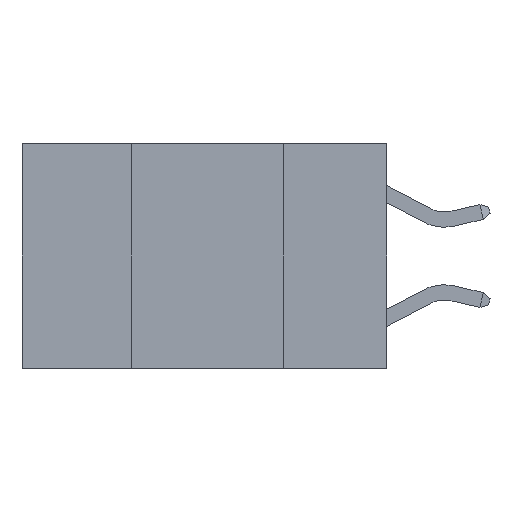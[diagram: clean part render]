
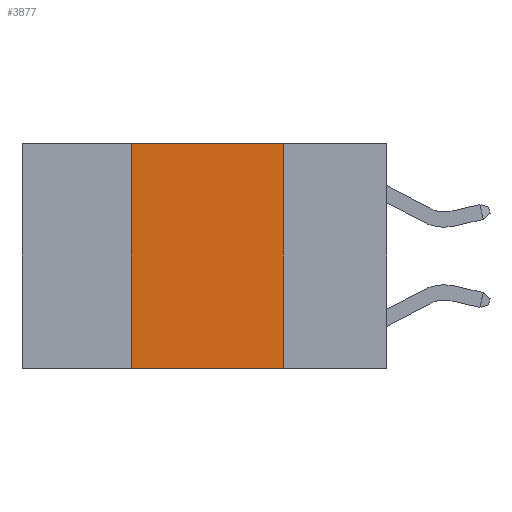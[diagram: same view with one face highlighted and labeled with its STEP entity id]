
A CAD part, left-side view. The second image highlights one B-rep face of the part: STEP entity #3877.
In plain terms, the highlighted planar face has unit normal (-1, 0, 0).
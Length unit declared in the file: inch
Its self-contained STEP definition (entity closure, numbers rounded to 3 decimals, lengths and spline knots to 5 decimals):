
#392 = VERTEX_POINT ( 'NONE', #10658 ) ;
#1095 = EDGE_LOOP ( 'NONE', ( #10278, #11160, #5317, #4137 ) ) ;
#2030 = CARTESIAN_POINT ( 'NONE',  ( 0., 0.42, 0. ) ) ;
#2975 = VECTOR ( 'NONE', #8717, 39.37008 ) ;
#3010 = CARTESIAN_POINT ( 'NONE',  ( 0., 0.6, 0. ) ) ;
#3042 = EDGE_CURVE ( 'NONE', #7221, #392, #9902, .T. ) ;
#3664 = CARTESIAN_POINT ( 'NONE',  ( 0., 0.6, -0.37 ) ) ;
#3715 = LINE ( 'NONE', #2030, #9602 ) ;
#3800 = DIRECTION ( 'NONE',  ( 1., 0., 0. ) ) ;
#3877 = ADVANCED_FACE ( 'NONE', ( #3980 ), #8273, .F. ) ;
#3980 = FACE_OUTER_BOUND ( 'NONE', #1095, .T. ) ;
#4137 = ORIENTED_EDGE ( 'NONE', *, *, #3042, .T. ) ;
#4946 = EDGE_CURVE ( 'NONE', #7221, #8030, #3715, .T. ) ;
#5032 = CARTESIAN_POINT ( 'NONE',  ( 0., 0.17, 0. ) ) ;
#5317 = ORIENTED_EDGE ( 'NONE', *, *, #4946, .F. ) ;
#5412 = CARTESIAN_POINT ( 'NONE',  ( 0., 0.42, 0. ) ) ;
#6104 = VECTOR ( 'NONE', #10630, 39.37008 ) ;
#6319 = CARTESIAN_POINT ( 'NONE',  ( 0., 0.17, 0. ) ) ;
#6638 = CARTESIAN_POINT ( 'NONE',  ( 0., 0.42, -0.37 ) ) ;
#6914 = CARTESIAN_POINT ( 'NONE',  ( 0., 0.6, 0. ) ) ;
#7056 = VERTEX_POINT ( 'NONE', #6319 ) ;
#7203 = DIRECTION ( 'NONE',  ( 0., 0., -1. ) ) ;
#7221 = VERTEX_POINT ( 'NONE', #6638 ) ;
#7633 = DIRECTION ( 'NONE',  ( 0., 0., -1. ) ) ;
#8030 = VERTEX_POINT ( 'NONE', #5412 ) ;
#8273 = PLANE ( 'NONE',  #10211 ) ;
#8407 = DIRECTION ( 'NONE',  ( 0., 0., 1. ) ) ;
#8659 = LINE ( 'NONE', #6914, #2975 ) ;
#8717 = DIRECTION ( 'NONE',  ( 0., -1., 0. ) ) ;
#8752 = EDGE_CURVE ( 'NONE', #8030, #7056, #8659, .T. ) ;
#9346 = LINE ( 'NONE', #5032, #9494 ) ;
#9494 = VECTOR ( 'NONE', #7633, 39.37008 ) ;
#9602 = VECTOR ( 'NONE', #8407, 39.37008 ) ;
#9902 = LINE ( 'NONE', #3664, #6104 ) ;
#10211 = AXIS2_PLACEMENT_3D ( 'NONE', #3010, #3800, #7203 ) ;
#10278 = ORIENTED_EDGE ( 'NONE', *, *, #11017, .F. ) ;
#10630 = DIRECTION ( 'NONE',  ( 0., -1., 0. ) ) ;
#10658 = CARTESIAN_POINT ( 'NONE',  ( 0., 0.17, -0.37 ) ) ;
#11017 = EDGE_CURVE ( 'NONE', #7056, #392, #9346, .T. ) ;
#11160 = ORIENTED_EDGE ( 'NONE', *, *, #8752, .F. ) ;
